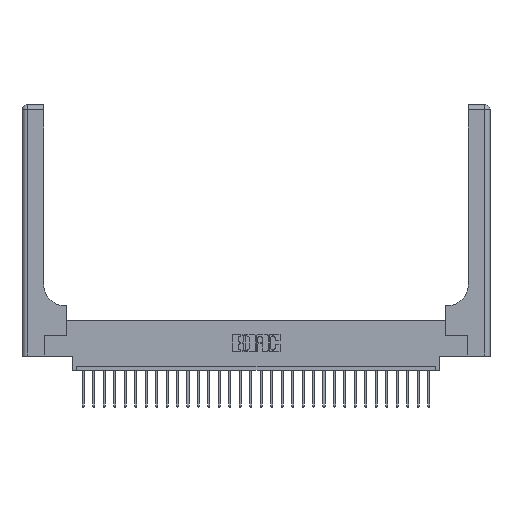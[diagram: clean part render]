
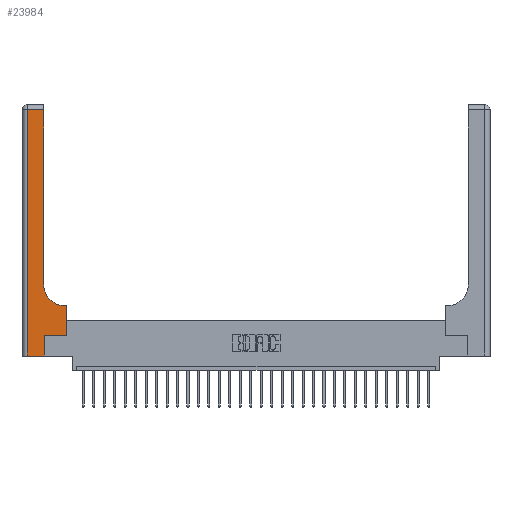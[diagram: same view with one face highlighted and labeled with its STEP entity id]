
A CAD part, top view. The second image highlights one B-rep face of the part: STEP entity #23984.
In plain terms, the highlighted planar face has unit normal (0, 0, 1).
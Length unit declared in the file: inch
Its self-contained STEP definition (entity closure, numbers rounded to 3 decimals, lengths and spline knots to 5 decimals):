
#161 = VERTEX_POINT ( 'NONE', #15761 ) ;
#1380 = EDGE_CURVE ( 'NONE', #8722, #15889, #6148, .T. ) ;
#1504 = DIRECTION ( 'NONE',  ( -1., 0., 0. ) ) ;
#1558 = VECTOR ( 'NONE', #14706, 39.37008 ) ;
#1943 = CARTESIAN_POINT ( 'NONE',  ( 0.265, 0., 0.37 ) ) ;
#2800 = ORIENTED_EDGE ( 'NONE', *, *, #21342, .T. ) ;
#3484 = VECTOR ( 'NONE', #5301, 39.37008 ) ;
#3639 = VECTOR ( 'NONE', #27016, 39.37008 ) ;
#3684 = VECTOR ( 'NONE', #14289, 39.37008 ) ;
#3756 = FACE_OUTER_BOUND ( 'NONE', #18323, .T. ) ;
#3940 = CARTESIAN_POINT ( 'NONE',  ( 0.26, 0.6, 0.37 ) ) ;
#4370 = CARTESIAN_POINT ( 'NONE',  ( 0.26, 2.94, 0.37 ) ) ;
#5301 = DIRECTION ( 'NONE',  ( 1., 0., 0. ) ) ;
#5372 = EDGE_CURVE ( 'NONE', #25405, #8722, #26293, .T. ) ;
#6108 = CARTESIAN_POINT ( 'NONE',  ( 0.265, 0.25, 0.37 ) ) ;
#6148 = LINE ( 'NONE', #26844, #3484 ) ;
#6798 = LINE ( 'NONE', #23360, #20752 ) ;
#6907 = VECTOR ( 'NONE', #20734, 39.37008 ) ;
#7154 = VERTEX_POINT ( 'NONE', #4370 ) ;
#7899 = VERTEX_POINT ( 'NONE', #21687 ) ;
#7913 = VERTEX_POINT ( 'NONE', #24019 ) ;
#8300 = EDGE_CURVE ( 'NONE', #7913, #22876, #21149, .T. ) ;
#8368 = ORIENTED_EDGE ( 'NONE', *, *, #23219, .T. ) ;
#8721 = AXIS2_PLACEMENT_3D ( 'NONE', #16195, #12080, #1504 ) ;
#8722 = VERTEX_POINT ( 'NONE', #24186 ) ;
#9806 = EDGE_CURVE ( 'NONE', #15889, #26806, #15764, .T. ) ;
#9865 = PLANE ( 'NONE',  #8721 ) ;
#10704 = CARTESIAN_POINT ( 'NONE',  ( 0.51, 0.85, 0.37 ) ) ;
#11941 = CARTESIAN_POINT ( 'NONE',  ( 0.51, 0.6, 0.37 ) ) ;
#12019 = CARTESIAN_POINT ( 'NONE',  ( 0., 2.94, 0.37 ) ) ;
#12080 = DIRECTION ( 'NONE',  ( 0., 0., -1. ) ) ;
#12264 = LINE ( 'NONE', #18225, #3639 ) ;
#14289 = DIRECTION ( 'NONE',  ( 0., -1., 0. ) ) ;
#14375 = ORIENTED_EDGE ( 'NONE', *, *, #19455, .T. ) ;
#14706 = DIRECTION ( 'NONE',  ( -1., 0., 0. ) ) ;
#15351 = CARTESIAN_POINT ( 'NONE',  ( 0.06, 2.94, 0.37 ) ) ;
#15761 = CARTESIAN_POINT ( 'NONE',  ( 0.528, 0.25, 0.37 ) ) ;
#15764 = LINE ( 'NONE', #27104, #22088 ) ;
#15889 = VERTEX_POINT ( 'NONE', #1943 ) ;
#15934 = ORIENTED_EDGE ( 'NONE', *, *, #1380, .T. ) ;
#16195 = CARTESIAN_POINT ( 'NONE',  ( 0., 3., 0.37 ) ) ;
#17695 = ORIENTED_EDGE ( 'NONE', *, *, #20575, .T. ) ;
#17923 = ORIENTED_EDGE ( 'NONE', *, *, #8300, .T. ) ;
#18225 = CARTESIAN_POINT ( 'NONE',  ( 0.26, 3., 0.37 ) ) ;
#18323 = EDGE_LOOP ( 'NONE', ( #17695, #23817, #21334, #15934, #20116, #2800, #8368, #17923, #14375 ) ) ;
#18740 = DIRECTION ( 'NONE',  ( 0., 1., 0. ) ) ;
#19455 = EDGE_CURVE ( 'NONE', #22876, #7899, #21310, .T. ) ;
#20116 = ORIENTED_EDGE ( 'NONE', *, *, #9806, .T. ) ;
#20575 = EDGE_CURVE ( 'NONE', #7899, #7154, #12264, .T. ) ;
#20734 = DIRECTION ( 'NONE',  ( 1., 0., 0. ) ) ;
#20752 = VECTOR ( 'NONE', #23455, 39.37008 ) ;
#21149 = LINE ( 'NONE', #3940, #1558 ) ;
#21288 = DIRECTION ( 'NONE',  ( 0., 0., -1. ) ) ;
#21310 = CIRCLE ( 'NONE', #26637, 0.25 ) ;
#21334 = ORIENTED_EDGE ( 'NONE', *, *, #5372, .T. ) ;
#21342 = EDGE_CURVE ( 'NONE', #26806, #161, #22548, .T. ) ;
#21687 = CARTESIAN_POINT ( 'NONE',  ( 0.26, 0.85, 0.37 ) ) ;
#22088 = VECTOR ( 'NONE', #18740, 39.37008 ) ;
#22113 = VECTOR ( 'NONE', #27263, 39.37008 ) ;
#22548 = LINE ( 'NONE', #27163, #6907 ) ;
#22660 = CARTESIAN_POINT ( 'NONE',  ( 0.06, 3., 0.37 ) ) ;
#22876 = VERTEX_POINT ( 'NONE', #11941 ) ;
#23007 = EDGE_CURVE ( 'NONE', #7154, #25405, #26422, .T. ) ;
#23219 = EDGE_CURVE ( 'NONE', #161, #7913, #6798, .T. ) ;
#23360 = CARTESIAN_POINT ( 'NONE',  ( 0.528, 0.25, 0.37 ) ) ;
#23455 = DIRECTION ( 'NONE',  ( 0., 1., 0. ) ) ;
#23817 = ORIENTED_EDGE ( 'NONE', *, *, #23007, .T. ) ;
#23984 = ADVANCED_FACE ( 'NONE', ( #3756 ), #9865, .F. ) ;
#24019 = CARTESIAN_POINT ( 'NONE',  ( 0.528, 0.6, 0.37 ) ) ;
#24186 = CARTESIAN_POINT ( 'NONE',  ( 0.06, 0., 0.37 ) ) ;
#25405 = VERTEX_POINT ( 'NONE', #15351 ) ;
#25587 = DIRECTION ( 'NONE',  ( 1., 0., 0. ) ) ;
#26293 = LINE ( 'NONE', #22660, #3684 ) ;
#26422 = LINE ( 'NONE', #12019, #22113 ) ;
#26637 = AXIS2_PLACEMENT_3D ( 'NONE', #10704, #21288, #25587 ) ;
#26806 = VERTEX_POINT ( 'NONE', #6108 ) ;
#26844 = CARTESIAN_POINT ( 'NONE',  ( 0., 0., 0.37 ) ) ;
#27016 = DIRECTION ( 'NONE',  ( 0., 1., 0. ) ) ;
#27104 = CARTESIAN_POINT ( 'NONE',  ( 0.265, 0., 0.37 ) ) ;
#27163 = CARTESIAN_POINT ( 'NONE',  ( 0.265, 0.25, 0.37 ) ) ;
#27263 = DIRECTION ( 'NONE',  ( -1., 0., 0. ) ) ;
